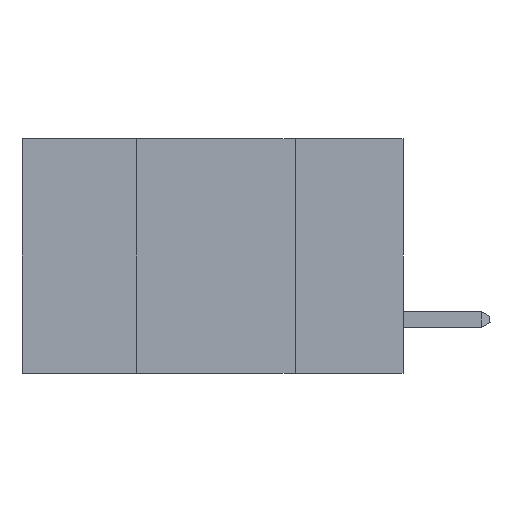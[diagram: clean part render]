
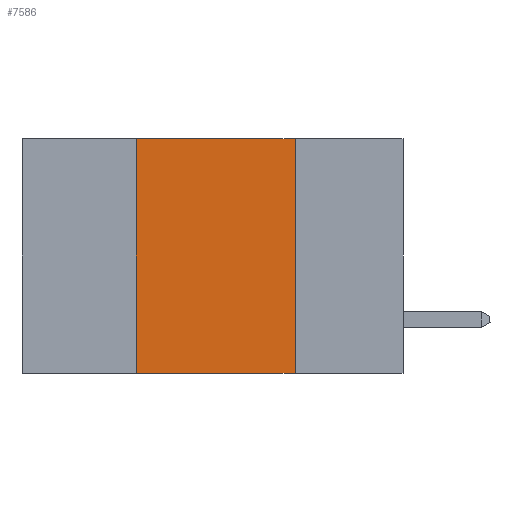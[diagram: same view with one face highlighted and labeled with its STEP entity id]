
A CAD part, left-side view. The second image highlights one B-rep face of the part: STEP entity #7586.
In plain terms, the highlighted planar face has unit normal (-1, 0, 0).
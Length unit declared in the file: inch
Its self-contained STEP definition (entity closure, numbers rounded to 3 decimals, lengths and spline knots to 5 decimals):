
#1 = AXIS2_PLACEMENT_3D ( 'NONE', #12935, #7682, #8751 ) ;
#492 = FACE_OUTER_BOUND ( 'NONE', #7176, .T. ) ;
#917 = VECTOR ( 'NONE', #6193, 39.37008 ) ;
#988 = DIRECTION ( 'NONE',  ( 0., -1., 0. ) ) ;
#1400 = CARTESIAN_POINT ( 'NONE',  ( 0., 0.42, -0.37 ) ) ;
#2086 = EDGE_CURVE ( 'NONE', #10394, #12101, #3143, .T. ) ;
#2587 = VECTOR ( 'NONE', #3150, 39.37008 ) ;
#2901 = LINE ( 'NONE', #4148, #2587 ) ;
#3143 = LINE ( 'NONE', #12267, #5669 ) ;
#3150 = DIRECTION ( 'NONE',  ( 0., 0., 1. ) ) ;
#4148 = CARTESIAN_POINT ( 'NONE',  ( 0., 0.42, 0. ) ) ;
#4269 = LINE ( 'NONE', #6945, #917 ) ;
#5072 = ORIENTED_EDGE ( 'NONE', *, *, #9992, .F. ) ;
#5608 = ORIENTED_EDGE ( 'NONE', *, *, #2086, .F. ) ;
#5669 = VECTOR ( 'NONE', #6198, 39.37008 ) ;
#6193 = DIRECTION ( 'NONE',  ( 0., -1., 0. ) ) ;
#6198 = DIRECTION ( 'NONE',  ( 0., 0., -1. ) ) ;
#6362 = CARTESIAN_POINT ( 'NONE',  ( 0., 0.17, 0. ) ) ;
#6945 = CARTESIAN_POINT ( 'NONE',  ( 0., 0.6, 0. ) ) ;
#7146 = EDGE_CURVE ( 'NONE', #8633, #12101, #9703, .T. ) ;
#7176 = EDGE_LOOP ( 'NONE', ( #5608, #5072, #7821, #7816 ) ) ;
#7228 = EDGE_CURVE ( 'NONE', #8633, #8708, #2901, .T. ) ;
#7586 = ADVANCED_FACE ( 'NONE', ( #492 ), #7731, .F. ) ;
#7632 = VECTOR ( 'NONE', #988, 39.37008 ) ;
#7682 = DIRECTION ( 'NONE',  ( 1., 0., 0. ) ) ;
#7731 = PLANE ( 'NONE',  #1 ) ;
#7816 = ORIENTED_EDGE ( 'NONE', *, *, #7146, .T. ) ;
#7821 = ORIENTED_EDGE ( 'NONE', *, *, #7228, .F. ) ;
#7962 = CARTESIAN_POINT ( 'NONE',  ( 0., 0.17, -0.37 ) ) ;
#8633 = VERTEX_POINT ( 'NONE', #1400 ) ;
#8708 = VERTEX_POINT ( 'NONE', #8975 ) ;
#8751 = DIRECTION ( 'NONE',  ( 0., 0., -1. ) ) ;
#8975 = CARTESIAN_POINT ( 'NONE',  ( 0., 0.42, 0. ) ) ;
#9166 = CARTESIAN_POINT ( 'NONE',  ( 0., 0.6, -0.37 ) ) ;
#9703 = LINE ( 'NONE', #9166, #7632 ) ;
#9992 = EDGE_CURVE ( 'NONE', #8708, #10394, #4269, .T. ) ;
#10394 = VERTEX_POINT ( 'NONE', #6362 ) ;
#12101 = VERTEX_POINT ( 'NONE', #7962 ) ;
#12267 = CARTESIAN_POINT ( 'NONE',  ( 0., 0.17, 0. ) ) ;
#12935 = CARTESIAN_POINT ( 'NONE',  ( 0., 0.6, 0. ) ) ;
